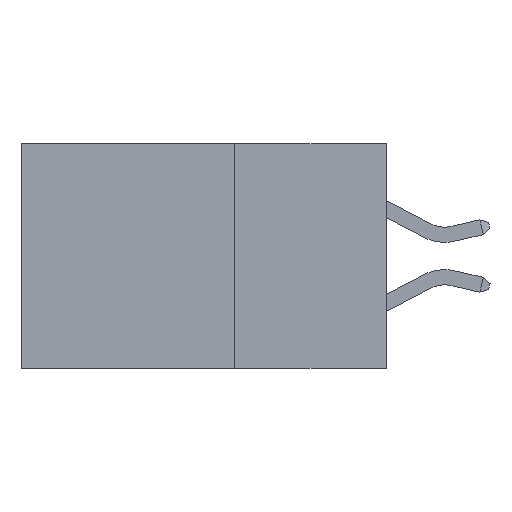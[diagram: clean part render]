
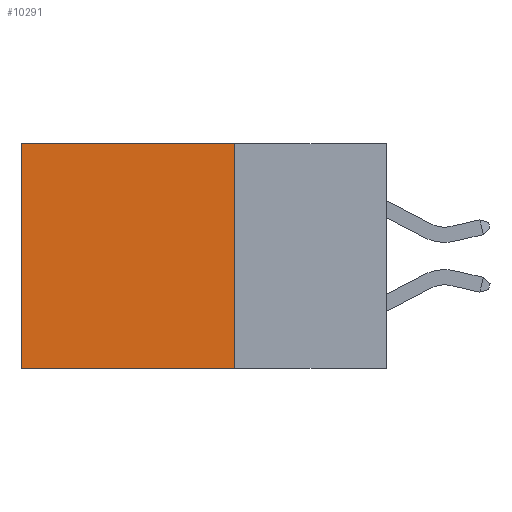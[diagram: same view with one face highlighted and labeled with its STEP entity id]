
A CAD part, left-side view. The second image highlights one B-rep face of the part: STEP entity #10291.
In plain terms, the highlighted planar face has unit normal (-1, 0, 0).
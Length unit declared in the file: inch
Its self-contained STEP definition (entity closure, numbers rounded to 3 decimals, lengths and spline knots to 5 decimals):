
#498 = VERTEX_POINT ( 'NONE', #15613 ) ;
#1543 = ORIENTED_EDGE ( 'NONE', *, *, #3528, .T. ) ;
#1954 = AXIS2_PLACEMENT_3D ( 'NONE', #6344, #9001, #3772 ) ;
#2086 = VECTOR ( 'NONE', #6956, 39.37008 ) ;
#2483 = CARTESIAN_POINT ( 'NONE',  ( 0.298, 0.6, 0. ) ) ;
#3528 = EDGE_CURVE ( 'NONE', #5929, #6345, #14610, .T. ) ;
#3772 = DIRECTION ( 'NONE',  ( 0., 0., -1. ) ) ;
#3938 = DIRECTION ( 'NONE',  ( 0., 0., -1. ) ) ;
#4013 = ORIENTED_EDGE ( 'NONE', *, *, #8768, .T. ) ;
#4791 = LINE ( 'NONE', #16091, #2086 ) ;
#5012 = PLANE ( 'NONE',  #1954 ) ;
#5124 = CARTESIAN_POINT ( 'NONE',  ( 0.298, 0.25, 0. ) ) ;
#5374 = DIRECTION ( 'NONE',  ( 0., 1., 0. ) ) ;
#5491 = ORIENTED_EDGE ( 'NONE', *, *, #12410, .F. ) ;
#5494 = FACE_OUTER_BOUND ( 'NONE', #12805, .T. ) ;
#5929 = VERTEX_POINT ( 'NONE', #13152 ) ;
#6344 = CARTESIAN_POINT ( 'NONE',  ( 0.298, 0.25, 0. ) ) ;
#6345 = VERTEX_POINT ( 'NONE', #9706 ) ;
#6498 = VERTEX_POINT ( 'NONE', #14201 ) ;
#6956 = DIRECTION ( 'NONE',  ( 0., 1., 0. ) ) ;
#7519 = VECTOR ( 'NONE', #3938, 39.37008 ) ;
#8300 = ORIENTED_EDGE ( 'NONE', *, *, #13436, .F. ) ;
#8768 = EDGE_CURVE ( 'NONE', #6498, #5929, #16336, .T. ) ;
#9001 = DIRECTION ( 'NONE',  ( 1., 0., 0. ) ) ;
#9706 = CARTESIAN_POINT ( 'NONE',  ( 0.298, 0.6, -0.37 ) ) ;
#9864 = VECTOR ( 'NONE', #15632, 39.37008 ) ;
#10291 = ADVANCED_FACE ( 'NONE', ( #5494 ), #5012, .F. ) ;
#12410 = EDGE_CURVE ( 'NONE', #6498, #498, #16226, .T. ) ;
#12805 = EDGE_LOOP ( 'NONE', ( #1543, #8300, #5491, #4013 ) ) ;
#13152 = CARTESIAN_POINT ( 'NONE',  ( 0.298, 0.6, 0. ) ) ;
#13436 = EDGE_CURVE ( 'NONE', #498, #6345, #4791, .T. ) ;
#13627 = VECTOR ( 'NONE', #5374, 39.37008 ) ;
#14201 = CARTESIAN_POINT ( 'NONE',  ( 0.298, 0.25, 0. ) ) ;
#14511 = CARTESIAN_POINT ( 'NONE',  ( 0.298, 0.25, 0. ) ) ;
#14610 = LINE ( 'NONE', #2483, #9864 ) ;
#15613 = CARTESIAN_POINT ( 'NONE',  ( 0.298, 0.25, -0.37 ) ) ;
#15632 = DIRECTION ( 'NONE',  ( 0., 0., -1. ) ) ;
#16091 = CARTESIAN_POINT ( 'NONE',  ( 0.298, 0.25, -0.37 ) ) ;
#16226 = LINE ( 'NONE', #5124, #7519 ) ;
#16336 = LINE ( 'NONE', #14511, #13627 ) ;
